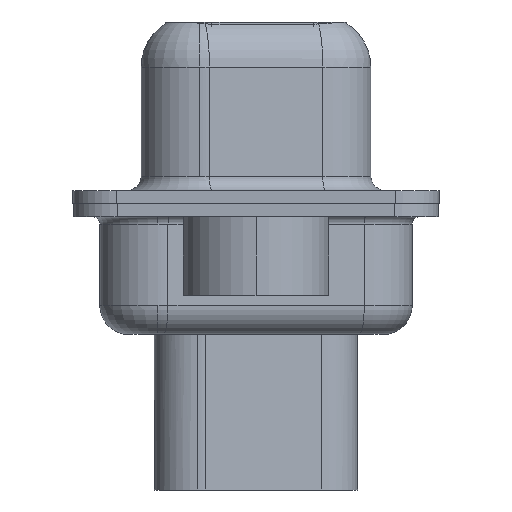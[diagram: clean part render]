
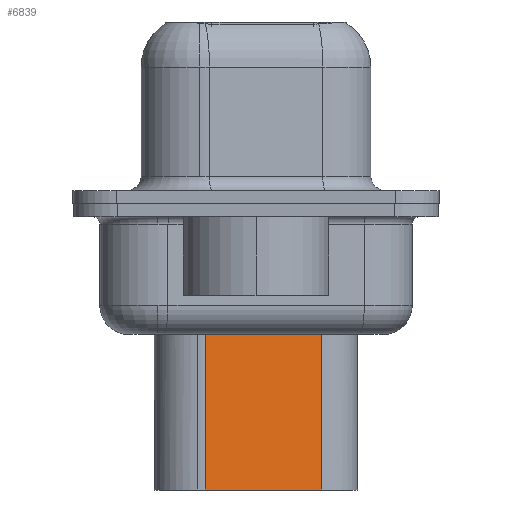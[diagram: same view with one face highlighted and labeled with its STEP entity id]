
A CAD part, left-side view. The second image highlights one B-rep face of the part: STEP entity #6839.
In plain terms, the highlighted planar face has unit normal (-0.985, -0.174, 0).
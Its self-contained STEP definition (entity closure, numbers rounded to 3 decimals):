
#16 = CARTESIAN_POINT ( 'NONE',  ( 4.519, 1.74, -3.975 ) ) ;
#885 = EDGE_CURVE ( 'NONE', #2683, #2987, #9924, .T. ) ;
#1109 = CARTESIAN_POINT ( 'NONE',  ( 5.224, -2.26, -9.85 ) ) ;
#1693 = DIRECTION ( 'NONE',  ( -0.985, -0.174, 0. ) ) ;
#2101 = VECTOR ( 'NONE', #14636, 1000. ) ;
#2450 = VERTEX_POINT ( 'NONE', #8196 ) ;
#2683 = VERTEX_POINT ( 'NONE', #4985 ) ;
#2987 = VERTEX_POINT ( 'NONE', #16 ) ;
#3189 = CARTESIAN_POINT ( 'NONE',  ( 4.519, 1.74, -3.1 ) ) ;
#3263 = CARTESIAN_POINT ( 'NONE',  ( 4.348, 2.709, -3.975 ) ) ;
#4049 = LINE ( 'NONE', #12106, #8230 ) ;
#4068 = LINE ( 'NONE', #10730, #10373 ) ;
#4090 = DIRECTION ( 'NONE',  ( 0.174, -0.985, 0. ) ) ;
#4429 = CARTESIAN_POINT ( 'NONE',  ( 4.519, 1.74, -9.85 ) ) ;
#4985 = CARTESIAN_POINT ( 'NONE',  ( 5.224, -2.26, -3.975 ) ) ;
#5031 = ORIENTED_EDGE ( 'NONE', *, *, #13918, .T. ) ;
#5059 = DIRECTION ( 'NONE',  ( 0., 0., -1. ) ) ;
#5920 = EDGE_CURVE ( 'NONE', #8288, #2450, #7794, .T. ) ;
#6839 = ADVANCED_FACE ( 'NONE', ( #8885 ), #13445, .T. ) ;
#7794 = LINE ( 'NONE', #4429, #10926 ) ;
#7896 = ORIENTED_EDGE ( 'NONE', *, *, #13365, .F. ) ;
#8196 = CARTESIAN_POINT ( 'NONE',  ( 4.519, 1.74, -9.85 ) ) ;
#8230 = VECTOR ( 'NONE', #8754, 1000. ) ;
#8288 = VERTEX_POINT ( 'NONE', #1109 ) ;
#8754 = DIRECTION ( 'NONE',  ( 0., 0., -1. ) ) ;
#8885 = FACE_OUTER_BOUND ( 'NONE', #10854, .T. ) ;
#8988 = DIRECTION ( 'NONE',  ( -0.174, 0.985, 0. ) ) ;
#9480 = ORIENTED_EDGE ( 'NONE', *, *, #885, .T. ) ;
#9924 = LINE ( 'NONE', #3263, #2101 ) ;
#10373 = VECTOR ( 'NONE', #5059, 1000. ) ;
#10730 = CARTESIAN_POINT ( 'NONE',  ( 5.224, -2.26, -3.1 ) ) ;
#10854 = EDGE_LOOP ( 'NONE', ( #7896, #9480, #5031, #10878 ) ) ;
#10878 = ORIENTED_EDGE ( 'NONE', *, *, #5920, .F. ) ;
#10926 = VECTOR ( 'NONE', #8988, 1000. ) ;
#12106 = CARTESIAN_POINT ( 'NONE',  ( 4.519, 1.74, -3.1 ) ) ;
#13327 = AXIS2_PLACEMENT_3D ( 'NONE', #3189, #1693, #4090 ) ;
#13365 = EDGE_CURVE ( 'NONE', #2683, #8288, #4068, .T. ) ;
#13445 = PLANE ( 'NONE',  #13327 ) ;
#13918 = EDGE_CURVE ( 'NONE', #2987, #2450, #4049, .T. ) ;
#14636 = DIRECTION ( 'NONE',  ( -0.174, 0.985, 0. ) ) ;
